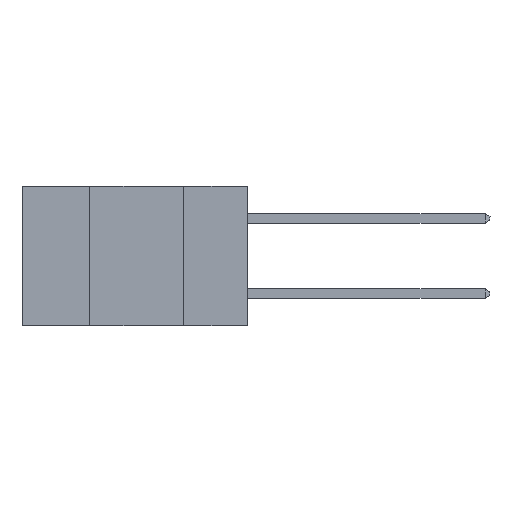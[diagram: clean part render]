
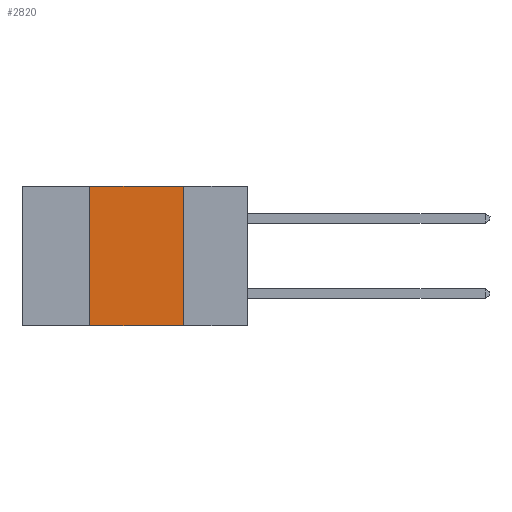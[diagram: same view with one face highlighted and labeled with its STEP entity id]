
A CAD part, left-side view. The second image highlights one B-rep face of the part: STEP entity #2820.
In plain terms, the highlighted planar face has unit normal (-1, 0, 0).
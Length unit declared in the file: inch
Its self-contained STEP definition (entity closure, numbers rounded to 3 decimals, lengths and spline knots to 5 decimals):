
#276 = DIRECTION ( 'NONE',  ( 0., 0., -1. ) ) ;
#522 = EDGE_LOOP ( 'NONE', ( #4104, #664, #6793, #9462 ) ) ;
#664 = ORIENTED_EDGE ( 'NONE', *, *, #5109, .F. ) ;
#1103 = DIRECTION ( 'NONE',  ( 0., -1., 0. ) ) ;
#1798 = VECTOR ( 'NONE', #9478, 39.37008 ) ;
#2232 = CARTESIAN_POINT ( 'NONE',  ( 0., 0.6, 0. ) ) ;
#2576 = DIRECTION ( 'NONE',  ( 0., 0., 1. ) ) ;
#2612 = CARTESIAN_POINT ( 'NONE',  ( 0., 0.17, 0. ) ) ;
#2820 = ADVANCED_FACE ( 'NONE', ( #6008 ), #9076, .F. ) ;
#2999 = VERTEX_POINT ( 'NONE', #6598 ) ;
#3315 = LINE ( 'NONE', #9424, #3549 ) ;
#3549 = VECTOR ( 'NONE', #2576, 39.37008 ) ;
#4007 = CARTESIAN_POINT ( 'NONE',  ( 0., 0.42, -0.37 ) ) ;
#4070 = VERTEX_POINT ( 'NONE', #6200 ) ;
#4104 = ORIENTED_EDGE ( 'NONE', *, *, #7254, .F. ) ;
#4134 = LINE ( 'NONE', #6407, #1798 ) ;
#4494 = DIRECTION ( 'NONE',  ( 0., -1., 0. ) ) ;
#4875 = LINE ( 'NONE', #7909, #5279 ) ;
#5109 = EDGE_CURVE ( 'NONE', #2999, #8942, #4875, .T. ) ;
#5137 = VECTOR ( 'NONE', #4494, 39.37008 ) ;
#5279 = VECTOR ( 'NONE', #1103, 39.37008 ) ;
#5460 = DIRECTION ( 'NONE',  ( 1., 0., 0. ) ) ;
#5692 = EDGE_CURVE ( 'NONE', #9250, #4070, #7633, .T. ) ;
#6008 = FACE_OUTER_BOUND ( 'NONE', #522, .T. ) ;
#6200 = CARTESIAN_POINT ( 'NONE',  ( 0., 0.17, -0.37 ) ) ;
#6407 = CARTESIAN_POINT ( 'NONE',  ( 0., 0.17, -0.37 ) ) ;
#6598 = CARTESIAN_POINT ( 'NONE',  ( 0., 0.42, 0. ) ) ;
#6754 = CARTESIAN_POINT ( 'NONE',  ( 0., 0.6, -0.37 ) ) ;
#6793 = ORIENTED_EDGE ( 'NONE', *, *, #7058, .F. ) ;
#7058 = EDGE_CURVE ( 'NONE', #9250, #2999, #3315, .T. ) ;
#7254 = EDGE_CURVE ( 'NONE', #8942, #4070, #4134, .T. ) ;
#7633 = LINE ( 'NONE', #6754, #5137 ) ;
#7909 = CARTESIAN_POINT ( 'NONE',  ( 0., 0.6, 0. ) ) ;
#8730 = AXIS2_PLACEMENT_3D ( 'NONE', #2232, #5460, #276 ) ;
#8942 = VERTEX_POINT ( 'NONE', #2612 ) ;
#9076 = PLANE ( 'NONE',  #8730 ) ;
#9250 = VERTEX_POINT ( 'NONE', #4007 ) ;
#9424 = CARTESIAN_POINT ( 'NONE',  ( 0., 0.42, -0.37 ) ) ;
#9462 = ORIENTED_EDGE ( 'NONE', *, *, #5692, .T. ) ;
#9478 = DIRECTION ( 'NONE',  ( 0., 0., -1. ) ) ;
